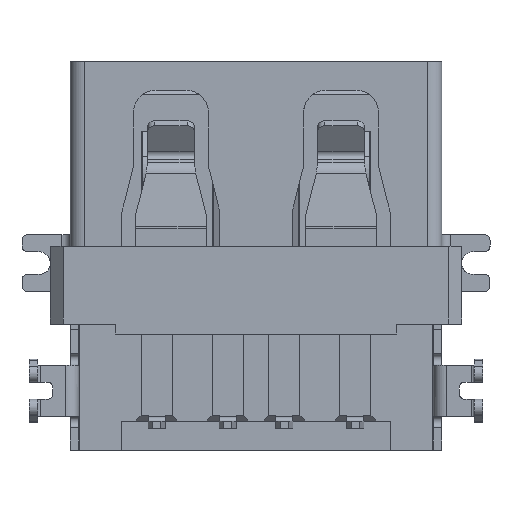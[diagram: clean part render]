
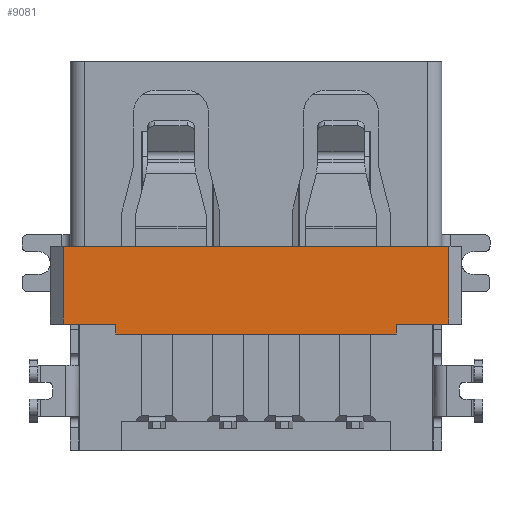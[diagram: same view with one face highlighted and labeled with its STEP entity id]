
A CAD part, front view. The second image highlights one B-rep face of the part: STEP entity #9081.
In plain terms, the highlighted planar face has unit normal (0, -1, 0).
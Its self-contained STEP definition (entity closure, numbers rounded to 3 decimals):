
#190 = CARTESIAN_POINT ( 'NONE',  ( -0.575, -6.12, 2.38 ) ) ;
#520 = CARTESIAN_POINT ( 'NONE',  ( 1.275, -6.12, -0.37 ) ) ;
#602 = DIRECTION ( 'NONE',  ( -1., 0., 0. ) ) ;
#1835 = VECTOR ( 'NONE', #11043, 1000. ) ;
#2429 = ORIENTED_EDGE ( 'NONE', *, *, #23124, .T. ) ;
#2466 = VECTOR ( 'NONE', #3215, 1000. ) ;
#3171 = VECTOR ( 'NONE', #20974, 1000. ) ;
#3215 = DIRECTION ( 'NONE',  ( 0., 0., 1. ) ) ;
#4330 = EDGE_CURVE ( 'NONE', #19637, #21898, #14631, .T. ) ;
#4425 = EDGE_CURVE ( 'NONE', #18880, #25680, #8853, .T. ) ;
#4666 = EDGE_LOOP ( 'NONE', ( #20641, #16859, #21744, #2429, #16600, #21432, #21361, #5247 ) ) ;
#5247 = ORIENTED_EDGE ( 'NONE', *, *, #4330, .F. ) ;
#5634 = FACE_OUTER_BOUND ( 'NONE', #4666, .T. ) ;
#7095 = LINE ( 'NONE', #26224, #22235 ) ;
#7374 = DIRECTION ( 'NONE',  ( -1., 0., 0. ) ) ;
#7696 = PLANE ( 'NONE',  #24883 ) ;
#8593 = LINE ( 'NONE', #15037, #12029 ) ;
#8828 = VECTOR ( 'NONE', #26381, 1000. ) ;
#8853 = LINE ( 'NONE', #23586, #1835 ) ;
#9081 = ADVANCED_FACE ( 'NONE', ( #5634 ), #7696, .F. ) ;
#9433 = EDGE_CURVE ( 'NONE', #25680, #24044, #20155, .T. ) ;
#9788 = CARTESIAN_POINT ( 'NONE',  ( -0.575, -6.12, -0.37 ) ) ;
#9923 = CARTESIAN_POINT ( 'NONE',  ( 1.275, -6.12, -0.545 ) ) ;
#10322 = VERTEX_POINT ( 'NONE', #16489 ) ;
#11043 = DIRECTION ( 'NONE',  ( -1., 0., 0. ) ) ;
#11537 = VECTOR ( 'NONE', #21663, 1000. ) ;
#12029 = VECTOR ( 'NONE', #602, 1000. ) ;
#12362 = DIRECTION ( 'NONE',  ( 0., 1., 0. ) ) ;
#12829 = VECTOR ( 'NONE', #16519, 1000. ) ;
#13117 = CARTESIAN_POINT ( 'NONE',  ( 6.225, -6.12, 2.38 ) ) ;
#14045 = LINE ( 'NONE', #9923, #12829 ) ;
#14146 = DIRECTION ( 'NONE',  ( 1., 0., 0. ) ) ;
#14425 = CARTESIAN_POINT ( 'NONE',  ( 6.225, -6.12, 0.83 ) ) ;
#14631 = LINE ( 'NONE', #23317, #3171 ) ;
#15037 = CARTESIAN_POINT ( 'NONE',  ( 6.225, -6.12, -0.37 ) ) ;
#16334 = EDGE_CURVE ( 'NONE', #10322, #16999, #18244, .T. ) ;
#16489 = CARTESIAN_POINT ( 'NONE',  ( 11.175, -6.12, -0.37 ) ) ;
#16519 = DIRECTION ( 'NONE',  ( 0., 0., -1. ) ) ;
#16600 = ORIENTED_EDGE ( 'NONE', *, *, #19767, .F. ) ;
#16848 = LINE ( 'NONE', #13117, #11537 ) ;
#16859 = ORIENTED_EDGE ( 'NONE', *, *, #9433, .F. ) ;
#16999 = VERTEX_POINT ( 'NONE', #23569 ) ;
#17801 = CARTESIAN_POINT ( 'NONE',  ( -0.575, -6.12, 0.83 ) ) ;
#18035 = CARTESIAN_POINT ( 'NONE',  ( 13.025, -6.12, -0.37 ) ) ;
#18244 = LINE ( 'NONE', #18390, #8828 ) ;
#18390 = CARTESIAN_POINT ( 'NONE',  ( 11.175, -6.12, -0.545 ) ) ;
#18486 = VERTEX_POINT ( 'NONE', #26016 ) ;
#18880 = VERTEX_POINT ( 'NONE', #520 ) ;
#19072 = CARTESIAN_POINT ( 'NONE',  ( 13.025, -6.12, 2.38 ) ) ;
#19637 = VERTEX_POINT ( 'NONE', #19072 ) ;
#19767 = EDGE_CURVE ( 'NONE', #16999, #18486, #7095, .T. ) ;
#20155 = LINE ( 'NONE', #17801, #2466 ) ;
#20641 = ORIENTED_EDGE ( 'NONE', *, *, #24029, .F. ) ;
#20974 = DIRECTION ( 'NONE',  ( 0., 0., -1. ) ) ;
#21361 = ORIENTED_EDGE ( 'NONE', *, *, #25120, .F. ) ;
#21432 = ORIENTED_EDGE ( 'NONE', *, *, #16334, .F. ) ;
#21663 = DIRECTION ( 'NONE',  ( 1., 0., 0. ) ) ;
#21744 = ORIENTED_EDGE ( 'NONE', *, *, #4425, .F. ) ;
#21898 = VERTEX_POINT ( 'NONE', #18035 ) ;
#22235 = VECTOR ( 'NONE', #7374, 1000. ) ;
#23124 = EDGE_CURVE ( 'NONE', #18880, #18486, #14045, .T. ) ;
#23317 = CARTESIAN_POINT ( 'NONE',  ( 13.025, -6.12, 0.83 ) ) ;
#23569 = CARTESIAN_POINT ( 'NONE',  ( 11.175, -6.12, -0.72 ) ) ;
#23586 = CARTESIAN_POINT ( 'NONE',  ( 6.225, -6.12, -0.37 ) ) ;
#24029 = EDGE_CURVE ( 'NONE', #24044, #19637, #16848, .T. ) ;
#24044 = VERTEX_POINT ( 'NONE', #190 ) ;
#24883 = AXIS2_PLACEMENT_3D ( 'NONE', #14425, #12362, #14146 ) ;
#25120 = EDGE_CURVE ( 'NONE', #21898, #10322, #8593, .T. ) ;
#25680 = VERTEX_POINT ( 'NONE', #9788 ) ;
#26016 = CARTESIAN_POINT ( 'NONE',  ( 1.275, -6.12, -0.72 ) ) ;
#26224 = CARTESIAN_POINT ( 'NONE',  ( 6.225, -6.12, -0.72 ) ) ;
#26381 = DIRECTION ( 'NONE',  ( 0., 0., -1. ) ) ;
